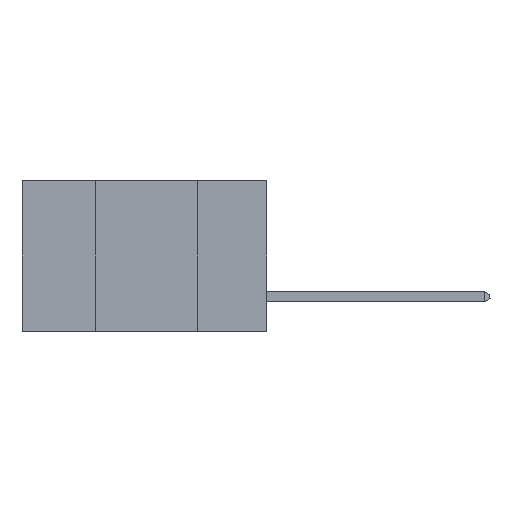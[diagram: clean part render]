
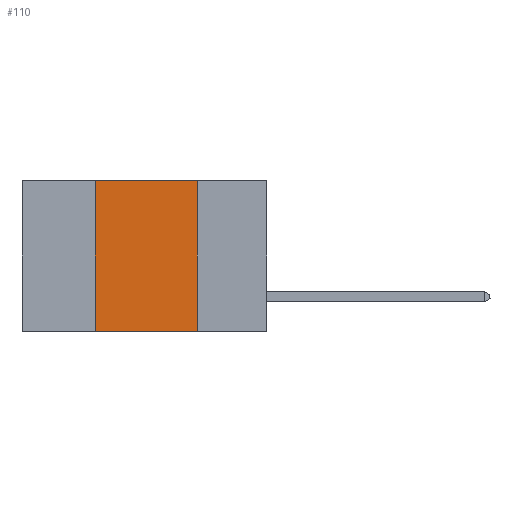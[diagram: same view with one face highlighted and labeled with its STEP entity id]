
A CAD part, left-side view. The second image highlights one B-rep face of the part: STEP entity #110.
In plain terms, the highlighted planar face has unit normal (-1, 0, 0).
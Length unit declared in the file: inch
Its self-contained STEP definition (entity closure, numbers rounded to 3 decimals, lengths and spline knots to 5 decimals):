
#110 = ADVANCED_FACE ( 'NONE', ( #7310 ), #3201, .F. ) ;
#403 = VERTEX_POINT ( 'NONE', #41490 ) ;
#2032 = CARTESIAN_POINT ( 'NONE',  ( 0., 0.6, -0.37 ) ) ;
#3201 = PLANE ( 'NONE',  #16885 ) ;
#7310 = FACE_OUTER_BOUND ( 'NONE', #21695, .T. ) ;
#8810 = VECTOR ( 'NONE', #35565, 39.37008 ) ;
#8931 = DIRECTION ( 'NONE',  ( 0., -1., 0. ) ) ;
#9029 = LINE ( 'NONE', #23244, #28974 ) ;
#9692 = DIRECTION ( 'NONE',  ( 0., 0., 1. ) ) ;
#10692 = DIRECTION ( 'NONE',  ( 0., 0., -1. ) ) ;
#11684 = EDGE_CURVE ( 'NONE', #22362, #19830, #9029, .T. ) ;
#12864 = VERTEX_POINT ( 'NONE', #28122 ) ;
#15741 = ORIENTED_EDGE ( 'NONE', *, *, #11684, .F. ) ;
#16885 = AXIS2_PLACEMENT_3D ( 'NONE', #27004, #44189, #33926 ) ;
#19312 = CARTESIAN_POINT ( 'NONE',  ( 0., 0.42, 0. ) ) ;
#19830 = VERTEX_POINT ( 'NONE', #19312 ) ;
#19868 = ORIENTED_EDGE ( 'NONE', *, *, #21674, .T. ) ;
#21674 = EDGE_CURVE ( 'NONE', #22362, #403, #22214, .T. ) ;
#21695 = EDGE_LOOP ( 'NONE', ( #22107, #38882, #15741, #19868 ) ) ;
#21718 = LINE ( 'NONE', #31813, #39604 ) ;
#22107 = ORIENTED_EDGE ( 'NONE', *, *, #26837, .F. ) ;
#22214 = LINE ( 'NONE', #2032, #38413 ) ;
#22362 = VERTEX_POINT ( 'NONE', #25751 ) ;
#23244 = CARTESIAN_POINT ( 'NONE',  ( 0., 0.42, 0. ) ) ;
#25751 = CARTESIAN_POINT ( 'NONE',  ( 0., 0.42, -0.37 ) ) ;
#26837 = EDGE_CURVE ( 'NONE', #12864, #403, #21718, .T. ) ;
#27004 = CARTESIAN_POINT ( 'NONE',  ( 0., 0.6, 0. ) ) ;
#28122 = CARTESIAN_POINT ( 'NONE',  ( 0., 0.17, 0. ) ) ;
#28803 = LINE ( 'NONE', #29246, #8810 ) ;
#28974 = VECTOR ( 'NONE', #9692, 39.37008 ) ;
#29246 = CARTESIAN_POINT ( 'NONE',  ( 0., 0.6, 0. ) ) ;
#31813 = CARTESIAN_POINT ( 'NONE',  ( 0., 0.17, 0. ) ) ;
#33926 = DIRECTION ( 'NONE',  ( 0., 0., -1. ) ) ;
#35565 = DIRECTION ( 'NONE',  ( 0., -1., 0. ) ) ;
#38413 = VECTOR ( 'NONE', #8931, 39.37008 ) ;
#38882 = ORIENTED_EDGE ( 'NONE', *, *, #40454, .F. ) ;
#39604 = VECTOR ( 'NONE', #10692, 39.37008 ) ;
#40454 = EDGE_CURVE ( 'NONE', #19830, #12864, #28803, .T. ) ;
#41490 = CARTESIAN_POINT ( 'NONE',  ( 0., 0.17, -0.37 ) ) ;
#44189 = DIRECTION ( 'NONE',  ( 1., 0., 0. ) ) ;
